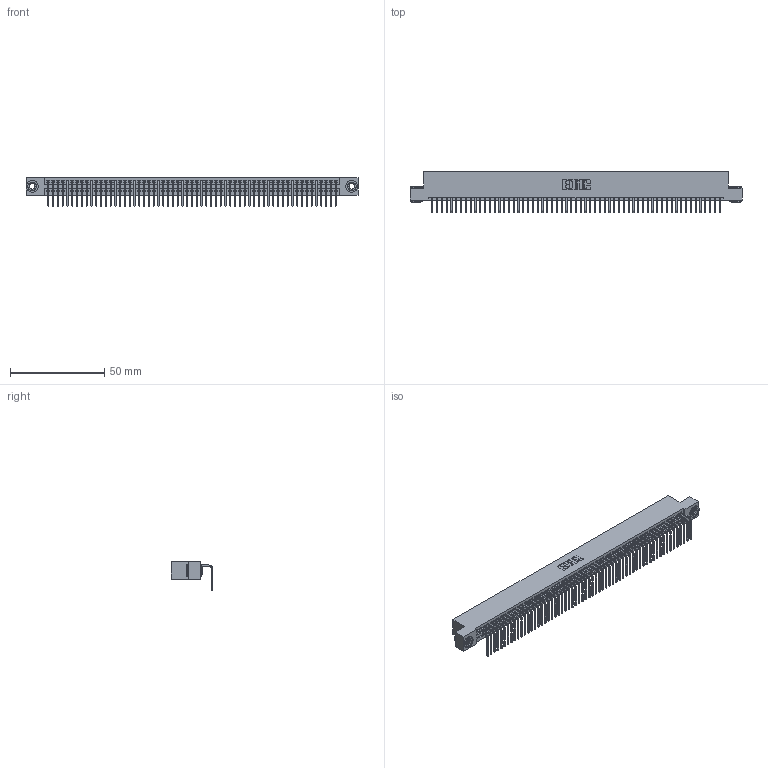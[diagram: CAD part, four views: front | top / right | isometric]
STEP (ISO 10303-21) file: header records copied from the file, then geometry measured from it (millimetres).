
FILE_DESCRIPTION (( 'STEP AP203' ), '1' );
FILE_NAME ('395-061-558-103.STEP', '2018-11-23T23:02:15', ( '' ), ( '' ), 'SwSTEP 2.0', 'SolidWorks 2016', '' );
FILE_SCHEMA (( 'CONFIG_CONTROL_DESIGN' ));
Length unit declared in the file: inch
Products named in the file (4): 395-061-558-103; 345-292-001_558 Tail - 2; 345 Part_Flush Mounting Lugs - 0.156 Dia-TH; 345-250-002_345-250-002-102
Assembly tree (64 placements, depth 2):
  395-061-558-103
    345 Part_Flush Mounting Lugs - 0.156 Dia-TH
    345-292-001_558 Tail - 2  x61
    345-250-002_345-250-002-102  x2
Bounding box: 176.15 x 21.83 x 15.37 mm (x, y, z)
Volume: 17109.1 mm3; surface area: 24403.4 mm2
Topology: 64 solids, 64 shells, 3824 faces, 11519 edges, 7594 vertices
Faces by surface type: plane 2652, cylinder 1164, cone 8
Entity records: 44086 total; most frequent: CARTESIAN_POINT 7614, ORIENTED_EDGE 7602, DIRECTION 6653, EDGE_CURVE 3801, LINE 3401, VECTOR 3401, VERTEX_POINT 2530, AXIS2_PLACEMENT_3D 1626
